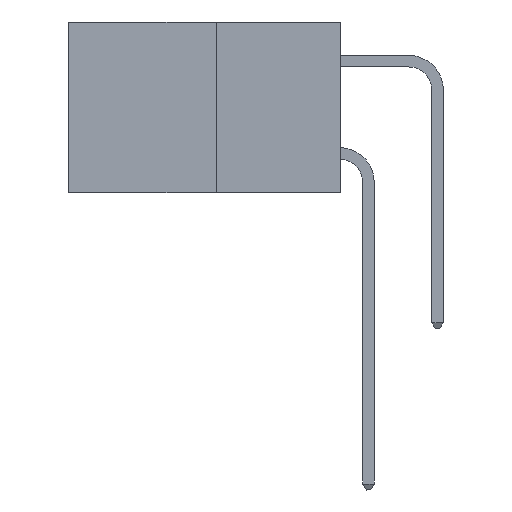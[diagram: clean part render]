
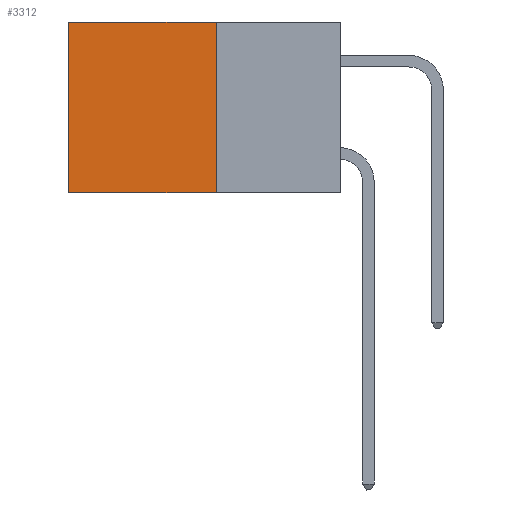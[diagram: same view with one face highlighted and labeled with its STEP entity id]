
A CAD part, left-side view. The second image highlights one B-rep face of the part: STEP entity #3312.
In plain terms, the highlighted planar face has unit normal (-1, 0, 0).
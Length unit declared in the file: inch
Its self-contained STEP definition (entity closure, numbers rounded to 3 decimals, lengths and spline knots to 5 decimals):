
#235 = VERTEX_POINT ( 'NONE', #2811 ) ;
#1228 = VECTOR ( 'NONE', #3046, 39.37008 ) ;
#2113 = CARTESIAN_POINT ( 'NONE',  ( 0.277, 0.27, -0.37 ) ) ;
#2139 = ORIENTED_EDGE ( 'NONE', *, *, #7234, .T. ) ;
#2278 = FACE_OUTER_BOUND ( 'NONE', #7878, .T. ) ;
#2303 = EDGE_CURVE ( 'NONE', #10637, #235, #9928, .T. ) ;
#2340 = VERTEX_POINT ( 'NONE', #5997 ) ;
#2368 = PLANE ( 'NONE',  #6306 ) ;
#2394 = CARTESIAN_POINT ( 'NONE',  ( 0.277, 0.27, -0.37 ) ) ;
#2811 = CARTESIAN_POINT ( 'NONE',  ( 0.277, 0.27, -0.37 ) ) ;
#2935 = LINE ( 'NONE', #7826, #9215 ) ;
#3046 = DIRECTION ( 'NONE',  ( 0., 1., 0. ) ) ;
#3118 = CARTESIAN_POINT ( 'NONE',  ( 0.277, 0.27, 0. ) ) ;
#3312 = ADVANCED_FACE ( 'NONE', ( #2278 ), #2368, .F. ) ;
#3551 = LINE ( 'NONE', #3118, #1228 ) ;
#3745 = DIRECTION ( 'NONE',  ( 0., 0., -1. ) ) ;
#4356 = EDGE_CURVE ( 'NONE', #235, #2340, #2935, .T. ) ;
#5997 = CARTESIAN_POINT ( 'NONE',  ( 0.277, 0.59, -0.37 ) ) ;
#6059 = VECTOR ( 'NONE', #3745, 39.37008 ) ;
#6194 = DIRECTION ( 'NONE',  ( 1., 0., 0. ) ) ;
#6306 = AXIS2_PLACEMENT_3D ( 'NONE', #2394, #6194, #9872 ) ;
#7234 = EDGE_CURVE ( 'NONE', #10637, #9771, #3551, .T. ) ;
#7612 = ORIENTED_EDGE ( 'NONE', *, *, #4356, .F. ) ;
#7696 = VECTOR ( 'NONE', #8122, 39.37008 ) ;
#7826 = CARTESIAN_POINT ( 'NONE',  ( 0.277, 0.27, -0.37 ) ) ;
#7878 = EDGE_LOOP ( 'NONE', ( #9595, #7612, #10359, #2139 ) ) ;
#7907 = CARTESIAN_POINT ( 'NONE',  ( 0.277, 0.59, 0. ) ) ;
#8122 = DIRECTION ( 'NONE',  ( 0., 0., -1. ) ) ;
#8499 = DIRECTION ( 'NONE',  ( 0., 1., 0. ) ) ;
#9215 = VECTOR ( 'NONE', #8499, 39.37008 ) ;
#9595 = ORIENTED_EDGE ( 'NONE', *, *, #9856, .T. ) ;
#9771 = VERTEX_POINT ( 'NONE', #7907 ) ;
#9856 = EDGE_CURVE ( 'NONE', #9771, #2340, #10554, .T. ) ;
#9872 = DIRECTION ( 'NONE',  ( 0., 0., -1. ) ) ;
#9928 = LINE ( 'NONE', #2113, #7696 ) ;
#10359 = ORIENTED_EDGE ( 'NONE', *, *, #2303, .F. ) ;
#10525 = CARTESIAN_POINT ( 'NONE',  ( 0.277, 0.59, -0.37 ) ) ;
#10554 = LINE ( 'NONE', #10525, #6059 ) ;
#10637 = VERTEX_POINT ( 'NONE', #10881 ) ;
#10881 = CARTESIAN_POINT ( 'NONE',  ( 0.277, 0.27, 0. ) ) ;
